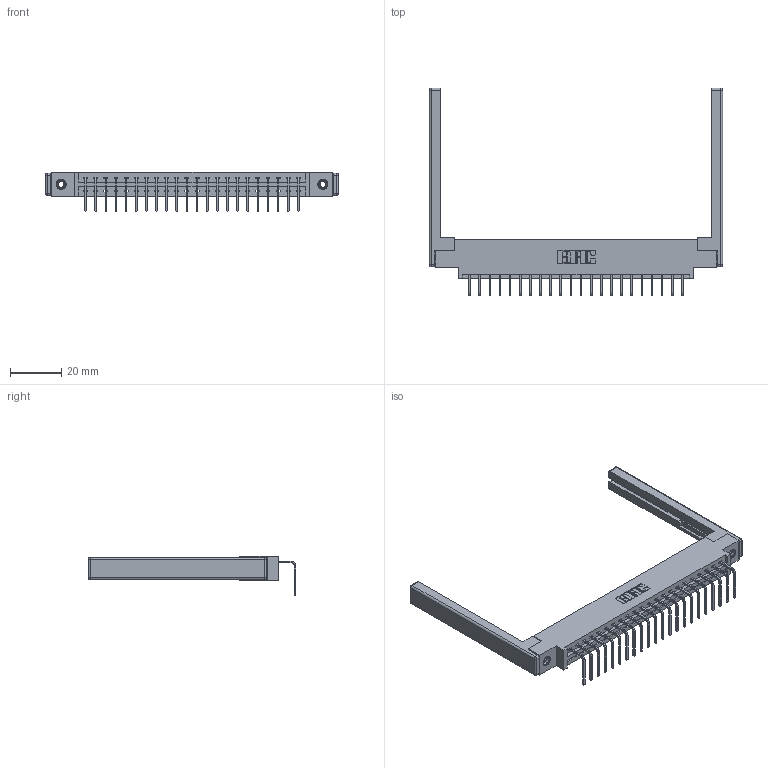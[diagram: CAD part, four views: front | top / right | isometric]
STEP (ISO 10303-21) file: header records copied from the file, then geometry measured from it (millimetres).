
FILE_DESCRIPTION (( 'STEP AP203' ), '1' );
FILE_NAME ('387-022-558-668.STEP', '2019-10-07T18:12:17', ( '' ), ( '' ), 'SwSTEP 2.0', 'SolidWorks 2016', '' );
FILE_SCHEMA (( 'CONFIG_CONTROL_DESIGN' ));
Length unit declared in the file: inch
Products named in the file (5): 345-292-001_558 Tail - 2; 337 Part_0.170 Offset - 0.156 Dia-TI; 387-022-558-668; 307-220-068; 345-250-001_345-250-001-102
Assembly tree (27 placements, depth 2):
  387-022-558-668
    337 Part_0.170 Offset - 0.156 Dia-TI
    345-292-001_558 Tail - 2  x22
    345-250-001_345-250-001-102  x2
    307-220-068  x2
Bounding box: 114.6 x 81.22 x 15.37 mm (x, y, z)
Volume: 16008 mm3; surface area: 16532.6 mm2
Topology: 27 solids, 27 shells, 1680 faces, 4981 edges, 3270 vertices
Faces by surface type: plane 1218, cylinder 438, cone 12, sphere 8, torus 4
Entity records: 21916 total; most frequent: CARTESIAN_POINT 3773, ORIENTED_EDGE 3720, DIRECTION 3290, EDGE_CURVE 1860, LINE 1682, VECTOR 1682, VERTEX_POINT 1230, AXIS2_PLACEMENT_3D 804
